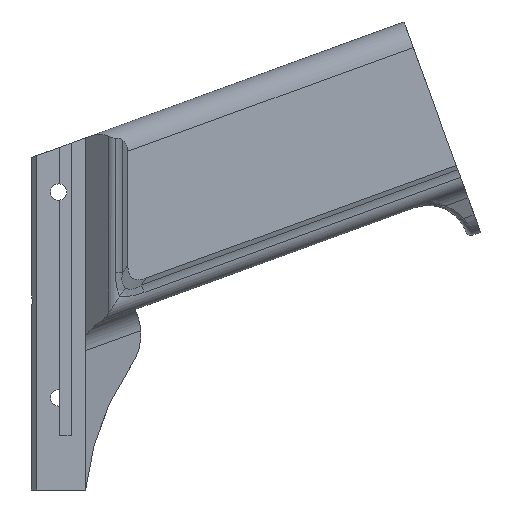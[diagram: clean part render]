
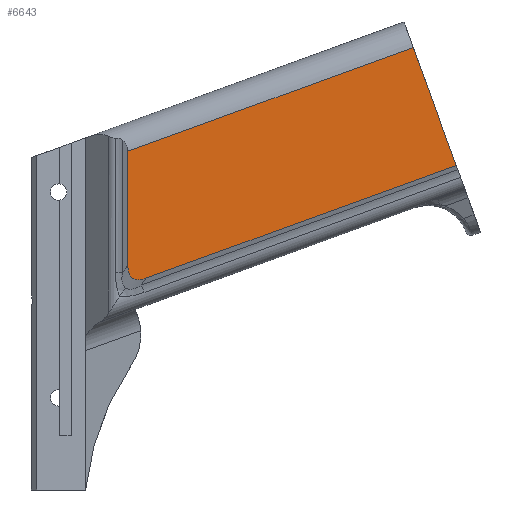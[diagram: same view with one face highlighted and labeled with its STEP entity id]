
A CAD part, left-side view. The second image highlights one B-rep face of the part: STEP entity #6643.
In plain terms, the highlighted planar face has unit normal (-1, 0, 0).
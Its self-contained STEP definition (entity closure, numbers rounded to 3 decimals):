
#80 = CARTESIAN_POINT ( 'NONE',  ( -11., -11.976, 31.433 ) ) ;
#147 = CARTESIAN_POINT ( 'NONE',  ( -11., -11.976, 31.433 ) ) ;
#401 = CARTESIAN_POINT ( 'NONE',  ( -11., -73.182, 48.297 ) ) ;
#759 = DIRECTION ( 'NONE',  ( 0., 0., -1. ) ) ;
#813 = CARTESIAN_POINT ( 'NONE',  ( -11., 0., 0. ) ) ;
#814 = DIRECTION ( 'NONE',  ( 0., -0.94, 0.342 ) ) ;
#926 = LINE ( 'NONE', #3816, #1333 ) ;
#1302 = VERTEX_POINT ( 'NONE', #80 ) ;
#1333 = VECTOR ( 'NONE', #2001, 1000. ) ;
#1585 = VERTEX_POINT ( 'NONE', #5050 ) ;
#1824 = DIRECTION ( 'NONE',  ( 0., 0., -1. ) ) ;
#1926 = ORIENTED_EDGE ( 'NONE', *, *, #2507, .T. ) ;
#2001 = DIRECTION ( 'NONE',  ( 0., 0.94, -0.342 ) ) ;
#2050 = EDGE_LOOP ( 'NONE', ( #1926, #2400, #6504, #2359, #2192 ) ) ;
#2058 = CARTESIAN_POINT ( 'NONE',  ( -11., -64.669, 71.685 ) ) ;
#2192 = ORIENTED_EDGE ( 'NONE', *, *, #5774, .T. ) ;
#2359 = ORIENTED_EDGE ( 'NONE', *, *, #5770, .T. ) ;
#2400 = ORIENTED_EDGE ( 'NONE', *, *, #5723, .T. ) ;
#2507 = EDGE_CURVE ( 'NONE', #6567, #3251, #6005, .T. ) ;
#2560 = LINE ( 'NONE', #6371, #4237 ) ;
#2638 = CARTESIAN_POINT ( 'NONE',  ( -11., -11.976, 29.127 ) ) ;
#2672 = VECTOR ( 'NONE', #7828, 1000. ) ;
#3251 = VERTEX_POINT ( 'NONE', #2058 ) ;
#3254 = CARTESIAN_POINT ( 'NONE',  ( -11., -15.331, 29.084 ) ) ;
#3282 = CARTESIAN_POINT ( 'NONE',  ( -11., -13.163, 28.295 ) ) ;
#3816 = CARTESIAN_POINT ( 'NONE',  ( -11., 15.474, 42.515 ) ) ;
#3870 = VECTOR ( 'NONE', #814, 1000. ) ;
#3950 = PLANE ( 'NONE',  #5393 ) ;
#4237 = VECTOR ( 'NONE', #759, 1000. ) ;
#4994 = VERTEX_POINT ( 'NONE', #3254 ) ;
#5050 = CARTESIAN_POINT ( 'NONE',  ( -11., -11.976, 52.506 ) ) ;
#5393 = AXIS2_PLACEMENT_3D ( 'NONE', #813, #7048, #1824 ) ;
#5510 = LINE ( 'NONE', #5789, #3870 ) ;
#5723 = EDGE_CURVE ( 'NONE', #3251, #1585, #926, .T. ) ;
#5739 = EDGE_CURVE ( 'NONE', #1585, #1302, #2560, .T. ) ;
#5770 = EDGE_CURVE ( 'NONE', #1302, #4994, #7944, .T. ) ;
#5774 = EDGE_CURVE ( 'NONE', #4994, #6567, #5510, .T. ) ;
#5789 = CARTESIAN_POINT ( 'NONE',  ( -11., 7.554, 20.755 ) ) ;
#6005 = LINE ( 'NONE', #401, #2672 ) ;
#6368 = FACE_OUTER_BOUND ( 'NONE', #2050, .T. ) ;
#6371 = CARTESIAN_POINT ( 'NONE',  ( -11., -11.976, 0. ) ) ;
#6504 = ORIENTED_EDGE ( 'NONE', *, *, #5739, .T. ) ;
#6567 = VERTEX_POINT ( 'NONE', #6840 ) ;
#6643 = ADVANCED_FACE ( 'NONE', ( #6368 ), #3950, .F. ) ;
#6840 = CARTESIAN_POINT ( 'NONE',  ( -11., -72.589, 49.925 ) ) ;
#7048 = DIRECTION ( 'NONE',  ( 1., 0., 0. ) ) ;
#7632 = CARTESIAN_POINT ( 'NONE',  ( -11., -15.331, 29.084 ) ) ;
#7828 = DIRECTION ( 'NONE',  ( 0., 0.342, 0.94 ) ) ;
#7944 =( BOUNDED_CURVE ( )  B_SPLINE_CURVE ( 3, ( #147, #2638, #3282, #7632 ),
 .UNSPECIFIED., .F., .T. ) 
 B_SPLINE_CURVE_WITH_KNOTS ( ( 4, 4 ),
 ( 2.72, 3.564 ),
 .UNSPECIFIED. ) 
 CURVE ( )  GEOMETRIC_REPRESENTATION_ITEM ( )  RATIONAL_B_SPLINE_CURVE ( ( 1., 0.942, 0.942, 1. ) ) 
 REPRESENTATION_ITEM ( '' )  );
